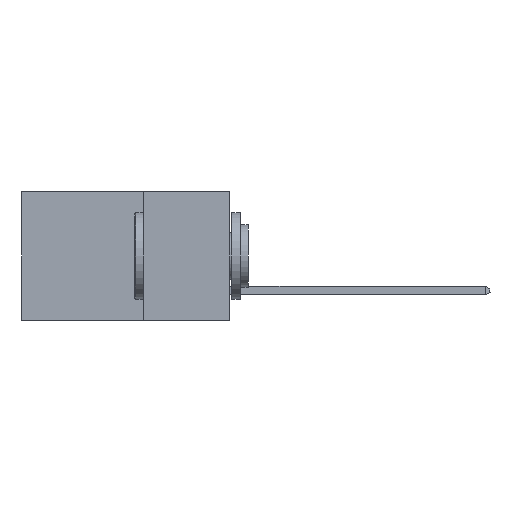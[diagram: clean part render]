
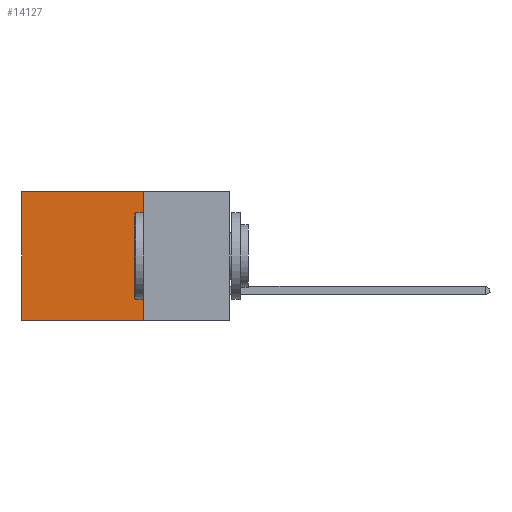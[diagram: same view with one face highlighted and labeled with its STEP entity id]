
A CAD part, left-side view. The second image highlights one B-rep face of the part: STEP entity #14127.
In plain terms, the highlighted planar face has unit normal (-1, 0, 0).
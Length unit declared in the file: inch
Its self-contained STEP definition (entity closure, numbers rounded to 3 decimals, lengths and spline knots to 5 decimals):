
#162 = VERTEX_POINT ( 'NONE', #12709 ) ;
#330 = LINE ( 'NONE', #15656, #7142 ) ;
#472 = LINE ( 'NONE', #7470, #18993 ) ;
#1146 = DIRECTION ( 'NONE',  ( 0., 0., -1. ) ) ;
#2307 = EDGE_CURVE ( 'NONE', #18958, #15166, #6868, .T. ) ;
#2422 = DIRECTION ( 'NONE',  ( 0., 0., -1. ) ) ;
#3230 = EDGE_CURVE ( 'NONE', #18958, #8435, #472, .T. ) ;
#3817 = DIRECTION ( 'NONE',  ( 0., 1., 0. ) ) ;
#4188 = EDGE_CURVE ( 'NONE', #15166, #162, #9219, .T. ) ;
#4711 = CARTESIAN_POINT ( 'NONE',  ( 0.298, 0.25, 0. ) ) ;
#6129 = DIRECTION ( 'NONE',  ( 0., 1., 0. ) ) ;
#6868 = LINE ( 'NONE', #14616, #7597 ) ;
#6886 = DIRECTION ( 'NONE',  ( 1., 0., 0. ) ) ;
#7142 = VECTOR ( 'NONE', #17013, 39.37008 ) ;
#7417 = CARTESIAN_POINT ( 'NONE',  ( 0.298, 0.6, 0. ) ) ;
#7470 = CARTESIAN_POINT ( 'NONE',  ( 0.298, 0.25, 0. ) ) ;
#7597 = VECTOR ( 'NONE', #1146, 39.37008 ) ;
#7812 = ORIENTED_EDGE ( 'NONE', *, *, #4188, .F. ) ;
#8435 = VERTEX_POINT ( 'NONE', #7417 ) ;
#8950 = FACE_OUTER_BOUND ( 'NONE', #11502, .T. ) ;
#9219 = LINE ( 'NONE', #18919, #9429 ) ;
#9429 = VECTOR ( 'NONE', #3817, 39.37008 ) ;
#10305 = CARTESIAN_POINT ( 'NONE',  ( 0.298, 0.25, -0.37 ) ) ;
#10527 = AXIS2_PLACEMENT_3D ( 'NONE', #17102, #6886, #2422 ) ;
#11502 = EDGE_LOOP ( 'NONE', ( #18485, #7812, #13473, #17559 ) ) ;
#12709 = CARTESIAN_POINT ( 'NONE',  ( 0.298, 0.6, -0.37 ) ) ;
#13473 = ORIENTED_EDGE ( 'NONE', *, *, #2307, .F. ) ;
#14127 = ADVANCED_FACE ( 'NONE', ( #8950 ), #17293, .F. ) ;
#14616 = CARTESIAN_POINT ( 'NONE',  ( 0.298, 0.25, 0. ) ) ;
#15166 = VERTEX_POINT ( 'NONE', #10305 ) ;
#15656 = CARTESIAN_POINT ( 'NONE',  ( 0.298, 0.6, 0. ) ) ;
#15928 = EDGE_CURVE ( 'NONE', #8435, #162, #330, .T. ) ;
#17013 = DIRECTION ( 'NONE',  ( 0., 0., -1. ) ) ;
#17102 = CARTESIAN_POINT ( 'NONE',  ( 0.298, 0.25, 0. ) ) ;
#17293 = PLANE ( 'NONE',  #10527 ) ;
#17559 = ORIENTED_EDGE ( 'NONE', *, *, #3230, .T. ) ;
#18485 = ORIENTED_EDGE ( 'NONE', *, *, #15928, .T. ) ;
#18919 = CARTESIAN_POINT ( 'NONE',  ( 0.298, 0.25, -0.37 ) ) ;
#18958 = VERTEX_POINT ( 'NONE', #4711 ) ;
#18993 = VECTOR ( 'NONE', #6129, 39.37008 ) ;
